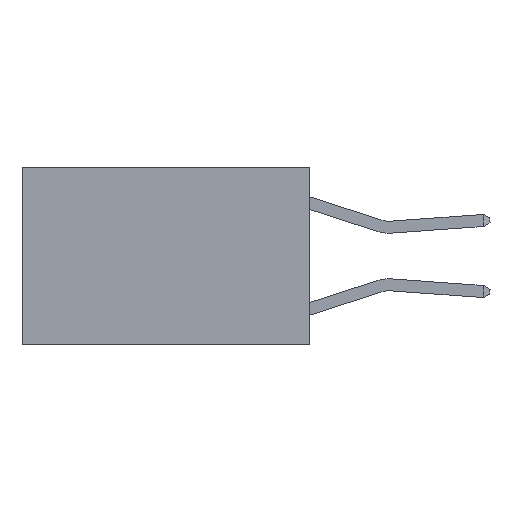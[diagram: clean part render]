
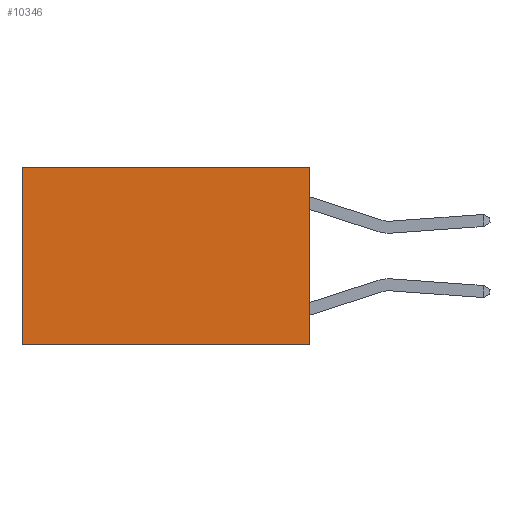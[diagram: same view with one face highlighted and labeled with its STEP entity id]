
A CAD part, left-side view. The second image highlights one B-rep face of the part: STEP entity #10346.
In plain terms, the highlighted planar face has unit normal (-1, 0, 0).
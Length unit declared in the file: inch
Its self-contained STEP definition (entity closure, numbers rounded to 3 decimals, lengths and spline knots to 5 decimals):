
#825 = VECTOR ( 'NONE', #13917, 39.37008 ) ;
#1045 = ORIENTED_EDGE ( 'NONE', *, *, #7029, .T. ) ;
#1067 = VERTEX_POINT ( 'NONE', #19060 ) ;
#1489 = CARTESIAN_POINT ( 'NONE',  ( 0.2625, 0., 0. ) ) ;
#1517 = ORIENTED_EDGE ( 'NONE', *, *, #2330, .F. ) ;
#1617 = LINE ( 'NONE', #18626, #17614 ) ;
#1660 = EDGE_CURVE ( 'NONE', #12658, #19384, #6823, .T. ) ;
#2130 = CARTESIAN_POINT ( 'NONE',  ( 0.2625, 0.6, -0.37 ) ) ;
#2330 = EDGE_CURVE ( 'NONE', #12658, #1067, #2993, .T. ) ;
#2575 = CARTESIAN_POINT ( 'NONE',  ( 0.2625, 0., 0. ) ) ;
#2993 = LINE ( 'NONE', #6386, #18551 ) ;
#3387 = LINE ( 'NONE', #12418, #825 ) ;
#3604 = DIRECTION ( 'NONE',  ( 0., 1., 0. ) ) ;
#4085 = DIRECTION ( 'NONE',  ( 1., 0., 0. ) ) ;
#5045 = ORIENTED_EDGE ( 'NONE', *, *, #13474, .F. ) ;
#6386 = CARTESIAN_POINT ( 'NONE',  ( 0.2625, 0., 0. ) ) ;
#6823 = LINE ( 'NONE', #18447, #10827 ) ;
#7029 = EDGE_CURVE ( 'NONE', #19384, #19370, #3387, .T. ) ;
#9449 = DIRECTION ( 'NONE',  ( 0., 1., 0. ) ) ;
#10105 = AXIS2_PLACEMENT_3D ( 'NONE', #2575, #4085, #14647 ) ;
#10346 = ADVANCED_FACE ( 'NONE', ( #12833 ), #13145, .F. ) ;
#10827 = VECTOR ( 'NONE', #9449, 39.37008 ) ;
#12418 = CARTESIAN_POINT ( 'NONE',  ( 0.2625, 0.6, 0. ) ) ;
#12658 = VERTEX_POINT ( 'NONE', #1489 ) ;
#12833 = FACE_OUTER_BOUND ( 'NONE', #18660, .T. ) ;
#13145 = PLANE ( 'NONE',  #10105 ) ;
#13474 = EDGE_CURVE ( 'NONE', #1067, #19370, #1617, .T. ) ;
#13917 = DIRECTION ( 'NONE',  ( 0., 0., -1. ) ) ;
#14647 = DIRECTION ( 'NONE',  ( 0., 0., -1. ) ) ;
#15390 = DIRECTION ( 'NONE',  ( 0., 0., -1. ) ) ;
#15697 = CARTESIAN_POINT ( 'NONE',  ( 0.2625, 0.6, 0. ) ) ;
#17519 = ORIENTED_EDGE ( 'NONE', *, *, #1660, .T. ) ;
#17614 = VECTOR ( 'NONE', #3604, 39.37008 ) ;
#18447 = CARTESIAN_POINT ( 'NONE',  ( 0.2625, 0., 0. ) ) ;
#18551 = VECTOR ( 'NONE', #15390, 39.37008 ) ;
#18626 = CARTESIAN_POINT ( 'NONE',  ( 0.2625, 0., -0.37 ) ) ;
#18660 = EDGE_LOOP ( 'NONE', ( #1045, #5045, #1517, #17519 ) ) ;
#19060 = CARTESIAN_POINT ( 'NONE',  ( 0.2625, 0., -0.37 ) ) ;
#19370 = VERTEX_POINT ( 'NONE', #2130 ) ;
#19384 = VERTEX_POINT ( 'NONE', #15697 ) ;
